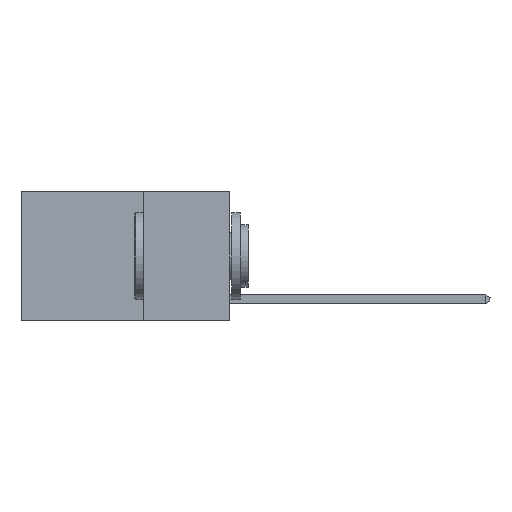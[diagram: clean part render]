
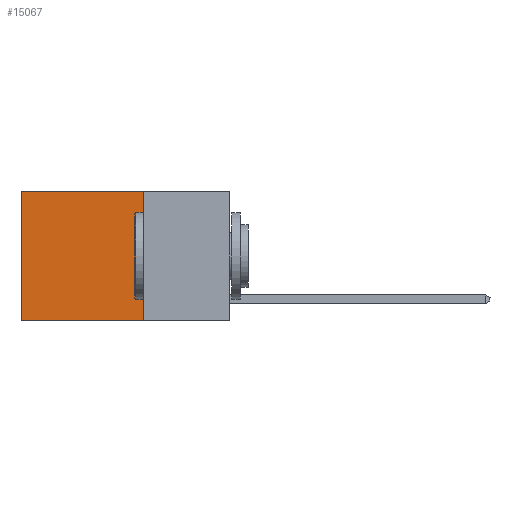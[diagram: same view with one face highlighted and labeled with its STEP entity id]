
A CAD part, left-side view. The second image highlights one B-rep face of the part: STEP entity #15067.
In plain terms, the highlighted planar face has unit normal (-1, 0, 0).
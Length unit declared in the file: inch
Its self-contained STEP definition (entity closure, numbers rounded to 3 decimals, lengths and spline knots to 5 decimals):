
#525 = CARTESIAN_POINT ( 'NONE',  ( 0.2625, 0.25, 0. ) ) ;
#1620 = CARTESIAN_POINT ( 'NONE',  ( 0.2625, 0.6, 0. ) ) ;
#2002 = CARTESIAN_POINT ( 'NONE',  ( 0.2625, 0.6, -0.37 ) ) ;
#2025 = DIRECTION ( 'NONE',  ( 0., 0., -1. ) ) ;
#2241 = EDGE_CURVE ( 'NONE', #23366, #4583, #8669, .T. ) ;
#2656 = EDGE_LOOP ( 'NONE', ( #2659, #27101, #20034, #4541 ) ) ;
#2659 = ORIENTED_EDGE ( 'NONE', *, *, #2241, .T. ) ;
#2750 = EDGE_CURVE ( 'NONE', #27462, #23366, #6288, .T. ) ;
#3837 = DIRECTION ( 'NONE',  ( 0., 0., -1. ) ) ;
#4541 = ORIENTED_EDGE ( 'NONE', *, *, #2750, .T. ) ;
#4583 = VERTEX_POINT ( 'NONE', #2002 ) ;
#5131 = LINE ( 'NONE', #24505, #11365 ) ;
#6288 = LINE ( 'NONE', #19569, #9628 ) ;
#6421 = FACE_OUTER_BOUND ( 'NONE', #2656, .T. ) ;
#6777 = DIRECTION ( 'NONE',  ( 0., 1., 0. ) ) ;
#8334 = DIRECTION ( 'NONE',  ( 0., 1., 0. ) ) ;
#8669 = LINE ( 'NONE', #1620, #13068 ) ;
#8764 = PLANE ( 'NONE',  #16136 ) ;
#9628 = VECTOR ( 'NONE', #8334, 39.37008 ) ;
#10837 = DIRECTION ( 'NONE',  ( 1., 0., 0. ) ) ;
#11365 = VECTOR ( 'NONE', #6777, 39.37008 ) ;
#11638 = CARTESIAN_POINT ( 'NONE',  ( 0.2625, 0.25, 0. ) ) ;
#13068 = VECTOR ( 'NONE', #3837, 39.37008 ) ;
#13758 = CARTESIAN_POINT ( 'NONE',  ( 0.2625, 0.6, 0. ) ) ;
#14750 = VECTOR ( 'NONE', #19035, 39.37008 ) ;
#14811 = EDGE_CURVE ( 'NONE', #17227, #4583, #5131, .T. ) ;
#15067 = ADVANCED_FACE ( 'NONE', ( #6421 ), #8764, .F. ) ;
#15440 = CARTESIAN_POINT ( 'NONE',  ( 0.2625, 0.25, 0. ) ) ;
#16136 = AXIS2_PLACEMENT_3D ( 'NONE', #15440, #10837, #2025 ) ;
#16239 = EDGE_CURVE ( 'NONE', #27462, #17227, #23019, .T. ) ;
#17007 = CARTESIAN_POINT ( 'NONE',  ( 0.2625, 0.25, -0.37 ) ) ;
#17227 = VERTEX_POINT ( 'NONE', #17007 ) ;
#19035 = DIRECTION ( 'NONE',  ( 0., 0., -1. ) ) ;
#19569 = CARTESIAN_POINT ( 'NONE',  ( 0.2625, 0.25, 0. ) ) ;
#20034 = ORIENTED_EDGE ( 'NONE', *, *, #16239, .F. ) ;
#23019 = LINE ( 'NONE', #11638, #14750 ) ;
#23366 = VERTEX_POINT ( 'NONE', #13758 ) ;
#24505 = CARTESIAN_POINT ( 'NONE',  ( 0.2625, 0.25, -0.37 ) ) ;
#27101 = ORIENTED_EDGE ( 'NONE', *, *, #14811, .F. ) ;
#27462 = VERTEX_POINT ( 'NONE', #525 ) ;
